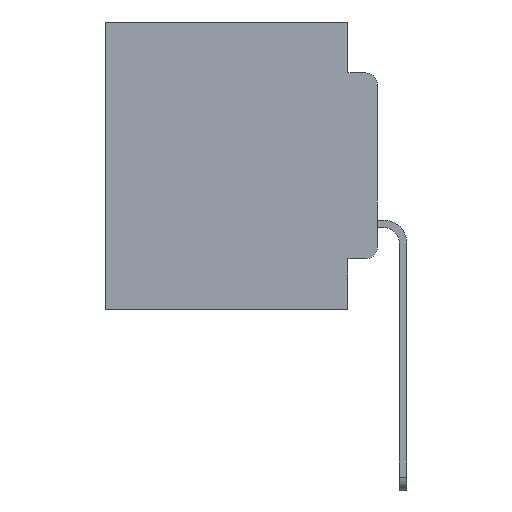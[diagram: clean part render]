
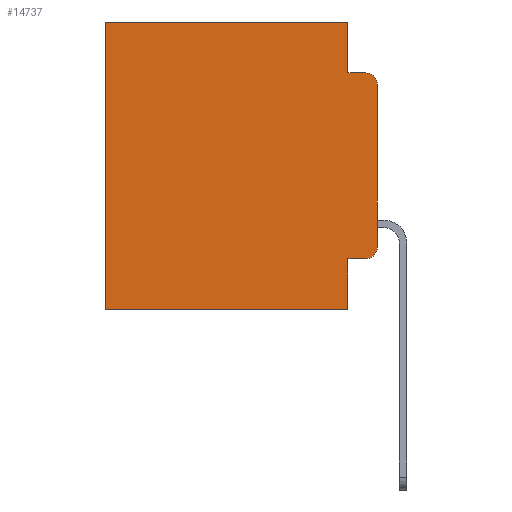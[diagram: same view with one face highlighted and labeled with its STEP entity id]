
A CAD part, left-side view. The second image highlights one B-rep face of the part: STEP entity #14737.
In plain terms, the highlighted planar face has unit normal (-1, 0, 0).
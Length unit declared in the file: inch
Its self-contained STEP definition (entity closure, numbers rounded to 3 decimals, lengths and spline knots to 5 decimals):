
#195 = VECTOR ( 'NONE', #11305, 39.37008 ) ;
#201 = EDGE_CURVE ( 'NONE', #11314, #26275, #6498, .T. ) ;
#332 = CARTESIAN_POINT ( 'NONE',  ( 0.298, 0.051, -0.0885 ) ) ;
#371 = DIRECTION ( 'NONE',  ( 0., 0., -1. ) ) ;
#1436 = ORIENTED_EDGE ( 'NONE', *, *, #11021, .T. ) ;
#1566 = VERTEX_POINT ( 'NONE', #10753 ) ;
#1794 = FACE_OUTER_BOUND ( 'NONE', #14513, .T. ) ;
#2231 = VERTEX_POINT ( 'NONE', #11376 ) ;
#3163 = CARTESIAN_POINT ( 'NONE',  ( 0.298, 0.051, -0.0885 ) ) ;
#3911 = DIRECTION ( 'NONE',  ( 1., 0., 0. ) ) ;
#3916 = CARTESIAN_POINT ( 'NONE',  ( 0.298, 0., 0. ) ) ;
#4574 = EDGE_CURVE ( 'NONE', #4952, #9604, #12230, .T. ) ;
#4952 = VERTEX_POINT ( 'NONE', #16223 ) ;
#4969 = EDGE_CURVE ( 'NONE', #25727, #24356, #14992, .T. ) ;
#5940 = ORIENTED_EDGE ( 'NONE', *, *, #21416, .F. ) ;
#6271 = DIRECTION ( 'NONE',  ( 0., 0., -1. ) ) ;
#6302 = CARTESIAN_POINT ( 'NONE',  ( 0.298, 0.051, 0. ) ) ;
#6498 = LINE ( 'NONE', #10677, #195 ) ;
#6513 = VECTOR ( 'NONE', #26560, 39.37008 ) ;
#7049 = DIRECTION ( 'NONE',  ( 0., 0., -1. ) ) ;
#7598 = CARTESIAN_POINT ( 'NONE',  ( 0.298, 0.02, -0.1085 ) ) ;
#7977 = VECTOR ( 'NONE', #371, 39.37008 ) ;
#8373 = VECTOR ( 'NONE', #22925, 39.37008 ) ;
#8620 = EDGE_CURVE ( 'NONE', #2231, #16508, #10892, .T. ) ;
#8888 = CARTESIAN_POINT ( 'NONE',  ( 0.298, 0.051, 0. ) ) ;
#9544 = CARTESIAN_POINT ( 'NONE',  ( 0.298, 0.02, -0.0885 ) ) ;
#9604 = VERTEX_POINT ( 'NONE', #24232 ) ;
#9862 = DIRECTION ( 'NONE',  ( 0., 0., -1. ) ) ;
#10444 = AXIS2_PLACEMENT_3D ( 'NONE', #7598, #23086, #9862 ) ;
#10601 = DIRECTION ( 'NONE',  ( -1., 0., 0. ) ) ;
#10677 = CARTESIAN_POINT ( 'NONE',  ( 0.298, 0., 0. ) ) ;
#10753 = CARTESIAN_POINT ( 'NONE',  ( 0.298, 0., -0.1085 ) ) ;
#10892 = LINE ( 'NONE', #21857, #21968 ) ;
#11021 = EDGE_CURVE ( 'NONE', #1566, #24356, #16006, .T. ) ;
#11305 = DIRECTION ( 'NONE',  ( 0., 1., 0. ) ) ;
#11314 = VERTEX_POINT ( 'NONE', #6302 ) ;
#11376 = CARTESIAN_POINT ( 'NONE',  ( 0.298, 0.051, -0.5 ) ) ;
#11930 = LINE ( 'NONE', #3916, #27431 ) ;
#12230 = CIRCLE ( 'NONE', #28016, 0.02 ) ;
#12466 = LINE ( 'NONE', #8888, #6513 ) ;
#12895 = CARTESIAN_POINT ( 'NONE',  ( 0.298, 0., 0. ) ) ;
#14096 = CARTESIAN_POINT ( 'NONE',  ( 0.298, 0.051, 0. ) ) ;
#14513 = EDGE_LOOP ( 'NONE', ( #5940, #1436, #16292, #18229, #20270, #27044, #28117, #26787, #27579, #20146 ) ) ;
#14565 = CARTESIAN_POINT ( 'NONE',  ( 0.298, 0.051, -0.4115 ) ) ;
#14737 = ADVANCED_FACE ( 'NONE', ( #1794 ), #17390, .F. ) ;
#14992 = LINE ( 'NONE', #332, #8373 ) ;
#16006 = CIRCLE ( 'NONE', #10444, 0.02 ) ;
#16223 = CARTESIAN_POINT ( 'NONE',  ( 0.298, 0.02, -0.4115 ) ) ;
#16292 = ORIENTED_EDGE ( 'NONE', *, *, #4969, .F. ) ;
#16498 = LINE ( 'NONE', #29062, #17176 ) ;
#16508 = VERTEX_POINT ( 'NONE', #23872 ) ;
#17176 = VECTOR ( 'NONE', #7049, 39.37008 ) ;
#17390 = PLANE ( 'NONE',  #21637 ) ;
#18077 = EDGE_CURVE ( 'NONE', #27457, #4952, #19393, .T. ) ;
#18229 = ORIENTED_EDGE ( 'NONE', *, *, #27803, .F. ) ;
#19393 = LINE ( 'NONE', #14565, #24531 ) ;
#19605 = DIRECTION ( 'NONE',  ( 0., 0., -1. ) ) ;
#20146 = ORIENTED_EDGE ( 'NONE', *, *, #4574, .T. ) ;
#20270 = ORIENTED_EDGE ( 'NONE', *, *, #201, .T. ) ;
#21056 = CARTESIAN_POINT ( 'NONE',  ( 0.298, 0.051, -0.4115 ) ) ;
#21207 = LINE ( 'NONE', #14096, #7977 ) ;
#21416 = EDGE_CURVE ( 'NONE', #1566, #9604, #11930, .T. ) ;
#21637 = AXIS2_PLACEMENT_3D ( 'NONE', #12895, #3911, #19605 ) ;
#21857 = CARTESIAN_POINT ( 'NONE',  ( 0.298, 0., -0.5 ) ) ;
#21968 = VECTOR ( 'NONE', #26237, 39.37008 ) ;
#22925 = DIRECTION ( 'NONE',  ( 0., -1., 0. ) ) ;
#23086 = DIRECTION ( 'NONE',  ( -1., 0., 0. ) ) ;
#23330 = DIRECTION ( 'NONE',  ( 0., -1., 0. ) ) ;
#23814 = CARTESIAN_POINT ( 'NONE',  ( 0.298, 0.02, -0.3915 ) ) ;
#23872 = CARTESIAN_POINT ( 'NONE',  ( 0.298, 0.473, -0.5 ) ) ;
#24232 = CARTESIAN_POINT ( 'NONE',  ( 0.298, 0., -0.3915 ) ) ;
#24356 = VERTEX_POINT ( 'NONE', #9544 ) ;
#24531 = VECTOR ( 'NONE', #23330, 39.37008 ) ;
#24900 = EDGE_CURVE ( 'NONE', #26275, #16508, #16498, .T. ) ;
#25140 = CARTESIAN_POINT ( 'NONE',  ( 0.298, 0.473, 0. ) ) ;
#25727 = VERTEX_POINT ( 'NONE', #3163 ) ;
#26029 = DIRECTION ( 'NONE',  ( 0., 0., -1. ) ) ;
#26237 = DIRECTION ( 'NONE',  ( 0., 1., 0. ) ) ;
#26275 = VERTEX_POINT ( 'NONE', #25140 ) ;
#26560 = DIRECTION ( 'NONE',  ( 0., 0., -1. ) ) ;
#26787 = ORIENTED_EDGE ( 'NONE', *, *, #26875, .F. ) ;
#26875 = EDGE_CURVE ( 'NONE', #27457, #2231, #21207, .T. ) ;
#27044 = ORIENTED_EDGE ( 'NONE', *, *, #24900, .T. ) ;
#27431 = VECTOR ( 'NONE', #6271, 39.37008 ) ;
#27457 = VERTEX_POINT ( 'NONE', #21056 ) ;
#27579 = ORIENTED_EDGE ( 'NONE', *, *, #18077, .T. ) ;
#27803 = EDGE_CURVE ( 'NONE', #11314, #25727, #12466, .T. ) ;
#28016 = AXIS2_PLACEMENT_3D ( 'NONE', #23814, #10601, #26029 ) ;
#28117 = ORIENTED_EDGE ( 'NONE', *, *, #8620, .F. ) ;
#29062 = CARTESIAN_POINT ( 'NONE',  ( 0.298, 0.473, 0. ) ) ;
